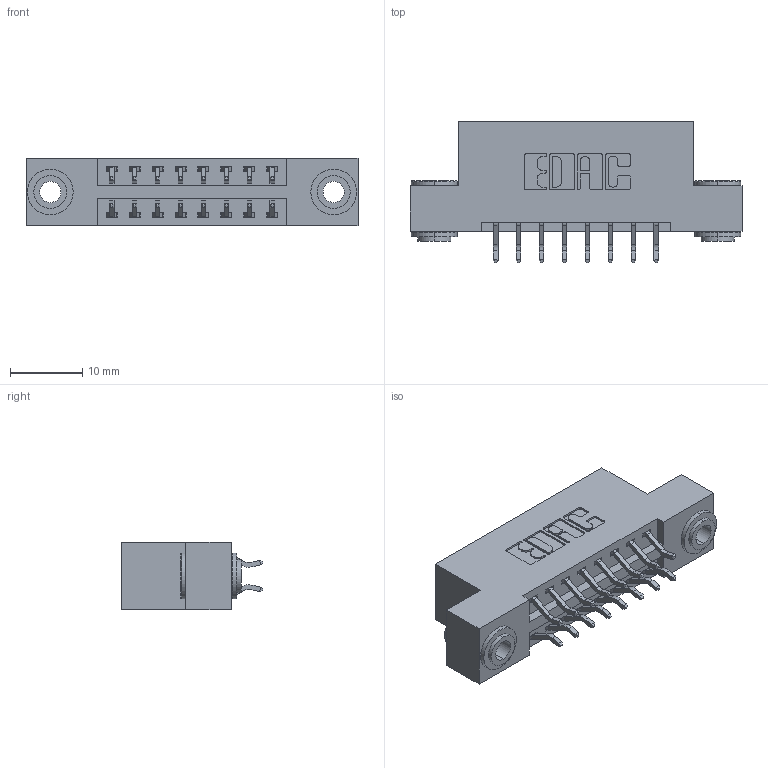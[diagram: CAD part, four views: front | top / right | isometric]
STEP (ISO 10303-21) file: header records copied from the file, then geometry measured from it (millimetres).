
FILE_DESCRIPTION (( 'STEP AP203' ), '1' );
FILE_NAME ('396-016-556-203.STEP', '2018-08-31T23:46:35', ( '' ), ( '' ), 'SwSTEP 2.0', 'SolidWorks 2016', '' );
FILE_SCHEMA (( 'CONFIG_CONTROL_DESIGN' ));
Length unit declared in the file: inch
Products named in the file (4): 345-250-002_345-250-002-102; 396-016-556-203; 346 Part_Flush Mounting Lugs - 0.156 Dia-TH; 345-292-001_556 Tail
Assembly tree (19 placements, depth 2):
  396-016-556-203
    346 Part_Flush Mounting Lugs - 0.156 Dia-TH
    345-292-001_556 Tail  x16
    345-250-002_345-250-002-102  x2
Bounding box: 45.97 x 19.57 x 9.4 mm (x, y, z)
Volume: 4237.7 mm3; surface area: 5490 mm2
Topology: 19 solids, 19 shells, 1088 faces, 3173 edges, 2090 vertices
Faces by surface type: plane 710, cylinder 370, cone 8
Entity records: 10668 total; most frequent: CARTESIAN_POINT 1795, ORIENTED_EDGE 1710, DIRECTION 1653, EDGE_CURVE 855, VECTOR 659, LINE 659, VERTEX_POINT 566, AXIS2_PLACEMENT_3D 497
